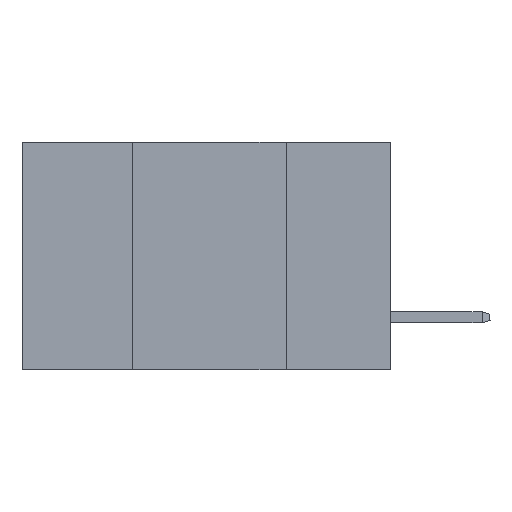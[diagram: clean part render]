
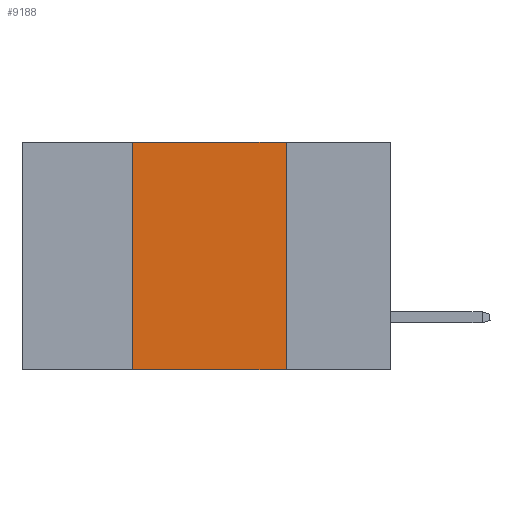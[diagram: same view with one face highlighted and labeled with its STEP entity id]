
A CAD part, left-side view. The second image highlights one B-rep face of the part: STEP entity #9188.
In plain terms, the highlighted planar face has unit normal (-1, 0, 0).
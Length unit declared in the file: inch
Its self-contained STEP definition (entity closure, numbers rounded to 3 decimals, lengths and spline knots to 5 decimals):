
#621 = LINE ( 'NONE', #2967, #3509 ) ;
#670 = VECTOR ( 'NONE', #851, 39.37008 ) ;
#851 = DIRECTION ( 'NONE',  ( 0., 0., -1. ) ) ;
#933 = LINE ( 'NONE', #7558, #8571 ) ;
#1472 = ORIENTED_EDGE ( 'NONE', *, *, #8073, .F. ) ;
#1735 = EDGE_CURVE ( 'NONE', #6973, #3268, #6089, .T. ) ;
#1790 = VERTEX_POINT ( 'NONE', #8047 ) ;
#1983 = DIRECTION ( 'NONE',  ( 1., 0., 0. ) ) ;
#2498 = ORIENTED_EDGE ( 'NONE', *, *, #5092, .T. ) ;
#2630 = PLANE ( 'NONE',  #5479 ) ;
#2637 = EDGE_LOOP ( 'NONE', ( #1472, #5866, #8171, #2498 ) ) ;
#2650 = CARTESIAN_POINT ( 'NONE',  ( 0., 0.42, -0.37 ) ) ;
#2967 = CARTESIAN_POINT ( 'NONE',  ( 0., 0.6, -0.37 ) ) ;
#3261 = CARTESIAN_POINT ( 'NONE',  ( 0., 0.17, 0. ) ) ;
#3268 = VERTEX_POINT ( 'NONE', #5056 ) ;
#3509 = VECTOR ( 'NONE', #4450, 39.37008 ) ;
#3834 = DIRECTION ( 'NONE',  ( 0., -1., 0. ) ) ;
#3856 = EDGE_CURVE ( 'NONE', #3268, #4869, #933, .T. ) ;
#4450 = DIRECTION ( 'NONE',  ( 0., -1., 0. ) ) ;
#4869 = VERTEX_POINT ( 'NONE', #3261 ) ;
#5056 = CARTESIAN_POINT ( 'NONE',  ( 0., 0.42, 0. ) ) ;
#5092 = EDGE_CURVE ( 'NONE', #6973, #1790, #621, .T. ) ;
#5479 = AXIS2_PLACEMENT_3D ( 'NONE', #8617, #1983, #7152 ) ;
#5866 = ORIENTED_EDGE ( 'NONE', *, *, #3856, .F. ) ;
#6089 = LINE ( 'NONE', #9266, #9567 ) ;
#6973 = VERTEX_POINT ( 'NONE', #2650 ) ;
#7064 = DIRECTION ( 'NONE',  ( 0., 0., 1. ) ) ;
#7152 = DIRECTION ( 'NONE',  ( 0., 0., -1. ) ) ;
#7525 = CARTESIAN_POINT ( 'NONE',  ( 0., 0.17, 0. ) ) ;
#7558 = CARTESIAN_POINT ( 'NONE',  ( 0., 0.6, 0. ) ) ;
#8047 = CARTESIAN_POINT ( 'NONE',  ( 0., 0.17, -0.37 ) ) ;
#8073 = EDGE_CURVE ( 'NONE', #4869, #1790, #8426, .T. ) ;
#8171 = ORIENTED_EDGE ( 'NONE', *, *, #1735, .F. ) ;
#8426 = LINE ( 'NONE', #7525, #670 ) ;
#8571 = VECTOR ( 'NONE', #3834, 39.37008 ) ;
#8617 = CARTESIAN_POINT ( 'NONE',  ( 0., 0.6, 0. ) ) ;
#8855 = FACE_OUTER_BOUND ( 'NONE', #2637, .T. ) ;
#9188 = ADVANCED_FACE ( 'NONE', ( #8855 ), #2630, .F. ) ;
#9266 = CARTESIAN_POINT ( 'NONE',  ( 0., 0.42, 0. ) ) ;
#9567 = VECTOR ( 'NONE', #7064, 39.37008 ) ;
